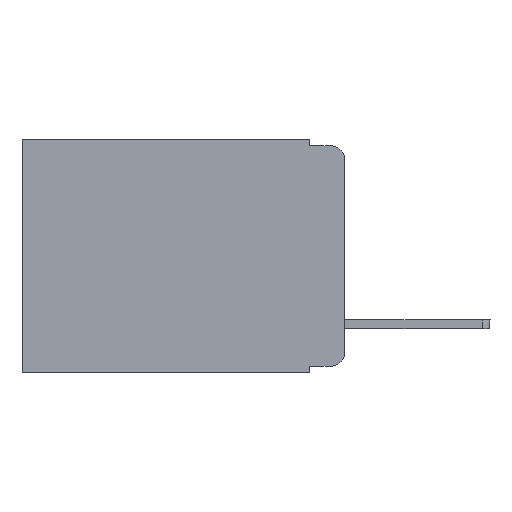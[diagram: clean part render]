
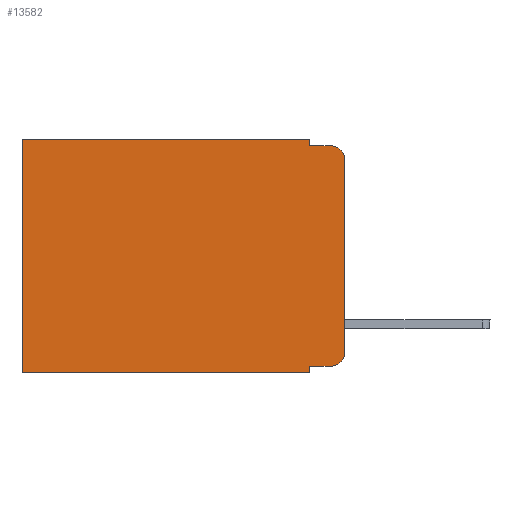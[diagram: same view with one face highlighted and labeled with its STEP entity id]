
A CAD part, left-side view. The second image highlights one B-rep face of the part: STEP entity #13582.
In plain terms, the highlighted planar face has unit normal (-1, 0, 0).
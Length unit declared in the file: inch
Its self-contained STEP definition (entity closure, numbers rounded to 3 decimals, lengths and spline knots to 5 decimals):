
#66 = CARTESIAN_POINT ( 'NONE',  ( 0.298, 0., -0.343 ) ) ;
#439 = CARTESIAN_POINT ( 'NONE',  ( 0.298, 0., 0. ) ) ;
#725 = EDGE_LOOP ( 'NONE', ( #3181, #14576, #3406, #4569, #20732, #12750, #12114, #19953, #5316, #15287 ) ) ;
#836 = LINE ( 'NONE', #11543, #17645 ) ;
#967 = CARTESIAN_POINT ( 'NONE',  ( 0.298, 0.473, 0. ) ) ;
#1193 = CARTESIAN_POINT ( 'NONE',  ( 0.298, 0.051, 0. ) ) ;
#1300 = VERTEX_POINT ( 'NONE', #1693 ) ;
#1402 = DIRECTION ( 'NONE',  ( 0., 1., 0. ) ) ;
#1693 = CARTESIAN_POINT ( 'NONE',  ( 0.298, 0.051, -0.333 ) ) ;
#1915 = EDGE_CURVE ( 'NONE', #14516, #15711, #2951, .T. ) ;
#2632 = LINE ( 'NONE', #5252, #18862 ) ;
#2951 = CIRCLE ( 'NONE', #12058, 0.02 ) ;
#3050 = CARTESIAN_POINT ( 'NONE',  ( 0.298, 0., -0.03 ) ) ;
#3181 = ORIENTED_EDGE ( 'NONE', *, *, #10226, .F. ) ;
#3406 = ORIENTED_EDGE ( 'NONE', *, *, #10109, .F. ) ;
#3715 = EDGE_CURVE ( 'NONE', #18046, #5823, #13887, .T. ) ;
#4243 = CARTESIAN_POINT ( 'NONE',  ( 0.298, 0.051, -0.01 ) ) ;
#4365 = CARTESIAN_POINT ( 'NONE',  ( 0.298, 0.02, -0.313 ) ) ;
#4475 = PLANE ( 'NONE',  #5664 ) ;
#4569 = ORIENTED_EDGE ( 'NONE', *, *, #19097, .F. ) ;
#4616 = DIRECTION ( 'NONE',  ( 0., 0., -1. ) ) ;
#4645 = DIRECTION ( 'NONE',  ( -1., 0., 0. ) ) ;
#4772 = CARTESIAN_POINT ( 'NONE',  ( 0.298, 0., 0. ) ) ;
#4804 = LINE ( 'NONE', #14326, #7308 ) ;
#5252 = CARTESIAN_POINT ( 'NONE',  ( 0.298, 0.051, 0. ) ) ;
#5316 = ORIENTED_EDGE ( 'NONE', *, *, #14539, .T. ) ;
#5461 = DIRECTION ( 'NONE',  ( 0., 0., -1. ) ) ;
#5663 = VECTOR ( 'NONE', #15061, 39.37008 ) ;
#5664 = AXIS2_PLACEMENT_3D ( 'NONE', #17484, #14206, #4616 ) ;
#5823 = VERTEX_POINT ( 'NONE', #14611 ) ;
#5933 = EDGE_CURVE ( 'NONE', #1300, #18046, #2632, .T. ) ;
#6065 = LINE ( 'NONE', #4772, #7816 ) ;
#6380 = VERTEX_POINT ( 'NONE', #14848 ) ;
#6539 = CARTESIAN_POINT ( 'NONE',  ( 0.298, 0.051, -0.333 ) ) ;
#7308 = VECTOR ( 'NONE', #7686, 39.37008 ) ;
#7686 = DIRECTION ( 'NONE',  ( 0., 0., -1. ) ) ;
#7816 = VECTOR ( 'NONE', #1402, 39.37008 ) ;
#8533 = VECTOR ( 'NONE', #9788, 39.37008 ) ;
#9172 = EDGE_CURVE ( 'NONE', #14255, #5823, #11845, .T. ) ;
#9788 = DIRECTION ( 'NONE',  ( 0., 1., 0. ) ) ;
#10109 = EDGE_CURVE ( 'NONE', #12407, #6380, #836, .T. ) ;
#10226 = EDGE_CURVE ( 'NONE', #20339, #15711, #18393, .T. ) ;
#11543 = CARTESIAN_POINT ( 'NONE',  ( 0.298, 0.051, -0.01 ) ) ;
#11704 = DIRECTION ( 'NONE',  ( 0., 0., -1. ) ) ;
#11716 = CARTESIAN_POINT ( 'NONE',  ( 0.298, 0., -0.313 ) ) ;
#11845 = LINE ( 'NONE', #18359, #20452 ) ;
#12058 = AXIS2_PLACEMENT_3D ( 'NONE', #4365, #4645, #14302 ) ;
#12114 = ORIENTED_EDGE ( 'NONE', *, *, #3715, .F. ) ;
#12407 = VERTEX_POINT ( 'NONE', #4243 ) ;
#12750 = ORIENTED_EDGE ( 'NONE', *, *, #9172, .T. ) ;
#12982 = VERTEX_POINT ( 'NONE', #1193 ) ;
#13311 = EDGE_CURVE ( 'NONE', #12982, #14255, #6065, .T. ) ;
#13582 = ADVANCED_FACE ( 'NONE', ( #19018 ), #4475, .F. ) ;
#13887 = LINE ( 'NONE', #66, #8533 ) ;
#14206 = DIRECTION ( 'NONE',  ( 1., 0., 0. ) ) ;
#14234 = DIRECTION ( 'NONE',  ( -1., 0., 0. ) ) ;
#14255 = VERTEX_POINT ( 'NONE', #967 ) ;
#14302 = DIRECTION ( 'NONE',  ( 0., 0., -1. ) ) ;
#14326 = CARTESIAN_POINT ( 'NONE',  ( 0.298, 0.051, 0. ) ) ;
#14516 = VERTEX_POINT ( 'NONE', #19625 ) ;
#14539 = EDGE_CURVE ( 'NONE', #1300, #14516, #15490, .T. ) ;
#14576 = ORIENTED_EDGE ( 'NONE', *, *, #14897, .T. ) ;
#14611 = CARTESIAN_POINT ( 'NONE',  ( 0.298, 0.473, -0.343 ) ) ;
#14848 = CARTESIAN_POINT ( 'NONE',  ( 0.298, 0.02, -0.01 ) ) ;
#14897 = EDGE_CURVE ( 'NONE', #20339, #6380, #17699, .T. ) ;
#14947 = DIRECTION ( 'NONE',  ( 0., -1., 0. ) ) ;
#15061 = DIRECTION ( 'NONE',  ( 0., 0., -1. ) ) ;
#15287 = ORIENTED_EDGE ( 'NONE', *, *, #1915, .T. ) ;
#15490 = LINE ( 'NONE', #6539, #16488 ) ;
#15507 = AXIS2_PLACEMENT_3D ( 'NONE', #19209, #14234, #20678 ) ;
#15711 = VERTEX_POINT ( 'NONE', #11716 ) ;
#16488 = VECTOR ( 'NONE', #14947, 39.37008 ) ;
#16496 = CARTESIAN_POINT ( 'NONE',  ( 0.298, 0.051, -0.343 ) ) ;
#17484 = CARTESIAN_POINT ( 'NONE',  ( 0.298, 0., 0. ) ) ;
#17645 = VECTOR ( 'NONE', #17723, 39.37008 ) ;
#17699 = CIRCLE ( 'NONE', #15507, 0.02 ) ;
#17723 = DIRECTION ( 'NONE',  ( 0., -1., 0. ) ) ;
#18046 = VERTEX_POINT ( 'NONE', #16496 ) ;
#18359 = CARTESIAN_POINT ( 'NONE',  ( 0.298, 0.473, 0. ) ) ;
#18393 = LINE ( 'NONE', #439, #5663 ) ;
#18862 = VECTOR ( 'NONE', #5461, 39.37008 ) ;
#19018 = FACE_OUTER_BOUND ( 'NONE', #725, .T. ) ;
#19097 = EDGE_CURVE ( 'NONE', #12982, #12407, #4804, .T. ) ;
#19209 = CARTESIAN_POINT ( 'NONE',  ( 0.298, 0.02, -0.03 ) ) ;
#19625 = CARTESIAN_POINT ( 'NONE',  ( 0.298, 0.02, -0.333 ) ) ;
#19953 = ORIENTED_EDGE ( 'NONE', *, *, #5933, .F. ) ;
#20339 = VERTEX_POINT ( 'NONE', #3050 ) ;
#20452 = VECTOR ( 'NONE', #11704, 39.37008 ) ;
#20678 = DIRECTION ( 'NONE',  ( 0., 0., -1. ) ) ;
#20732 = ORIENTED_EDGE ( 'NONE', *, *, #13311, .T. ) ;
